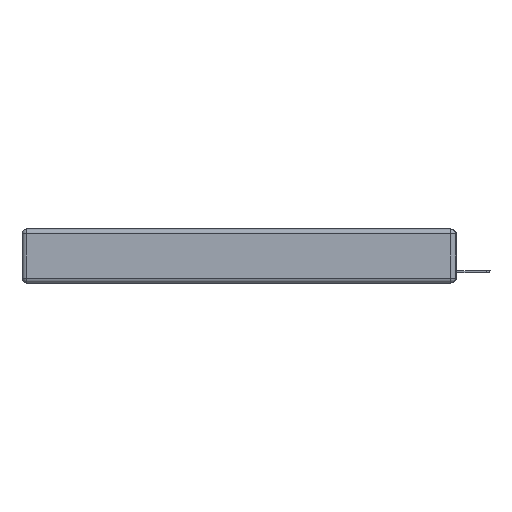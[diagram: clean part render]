
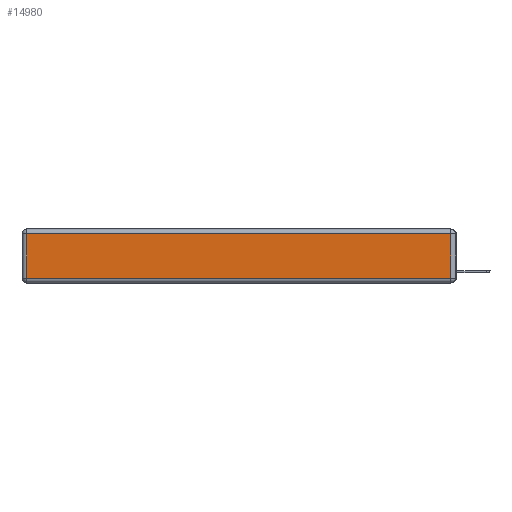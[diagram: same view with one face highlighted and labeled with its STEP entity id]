
A CAD part, left-side view. The second image highlights one B-rep face of the part: STEP entity #14980.
In plain terms, the highlighted planar face has unit normal (-1, 0, 0).
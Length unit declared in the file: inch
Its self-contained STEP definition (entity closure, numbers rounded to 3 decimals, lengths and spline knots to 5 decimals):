
#1404 = LINE ( 'NONE', #7475, #23342 ) ;
#1408 = DIRECTION ( 'NONE',  ( 0., 0., 1. ) ) ;
#1484 = VECTOR ( 'NONE', #13200, 39.37008 ) ;
#1834 = VERTEX_POINT ( 'NONE', #18658 ) ;
#2501 = DIRECTION ( 'NONE',  ( 0., 1., 0. ) ) ;
#3353 = ORIENTED_EDGE ( 'NONE', *, *, #20016, .T. ) ;
#4630 = VERTEX_POINT ( 'NONE', #9718 ) ;
#4944 = FACE_OUTER_BOUND ( 'NONE', #18767, .T. ) ;
#5005 = VECTOR ( 'NONE', #15818, 39.37008 ) ;
#7475 = CARTESIAN_POINT ( 'NONE',  ( 0., 0., -0.313 ) ) ;
#7671 = CARTESIAN_POINT ( 'NONE',  ( 0., 2.75, -0.03 ) ) ;
#8094 = ORIENTED_EDGE ( 'NONE', *, *, #8799, .T. ) ;
#8616 = CARTESIAN_POINT ( 'NONE',  ( 0., 0., -0.343 ) ) ;
#8799 = EDGE_CURVE ( 'NONE', #4630, #20863, #1404, .T. ) ;
#9718 = CARTESIAN_POINT ( 'NONE',  ( 0., 2.72, -0.313 ) ) ;
#12236 = DIRECTION ( 'NONE',  ( -1., 0., 0. ) ) ;
#12781 = VERTEX_POINT ( 'NONE', #13892 ) ;
#13046 = LINE ( 'NONE', #18549, #1484 ) ;
#13200 = DIRECTION ( 'NONE',  ( 0., 0., 1. ) ) ;
#13315 = ORIENTED_EDGE ( 'NONE', *, *, #15921, .T. ) ;
#13892 = CARTESIAN_POINT ( 'NONE',  ( 0., 2.72, -0.03 ) ) ;
#14158 = AXIS2_PLACEMENT_3D ( 'NONE', #8616, #12236, #1408 ) ;
#14569 = DIRECTION ( 'NONE',  ( 0., -1., 0. ) ) ;
#14980 = ADVANCED_FACE ( 'NONE', ( #4944 ), #19555, .T. ) ;
#15818 = DIRECTION ( 'NONE',  ( 0., 0., -1. ) ) ;
#15921 = EDGE_CURVE ( 'NONE', #20863, #1834, #13046, .T. ) ;
#16050 = CARTESIAN_POINT ( 'NONE',  ( 0., 2.72, -0.343 ) ) ;
#18222 = ORIENTED_EDGE ( 'NONE', *, *, #19063, .T. ) ;
#18278 = LINE ( 'NONE', #7671, #18864 ) ;
#18549 = CARTESIAN_POINT ( 'NONE',  ( 0., 0.03, -0.343 ) ) ;
#18658 = CARTESIAN_POINT ( 'NONE',  ( 0., 0.03, -0.03 ) ) ;
#18767 = EDGE_LOOP ( 'NONE', ( #8094, #13315, #18222, #3353 ) ) ;
#18864 = VECTOR ( 'NONE', #2501, 39.37008 ) ;
#19063 = EDGE_CURVE ( 'NONE', #1834, #12781, #18278, .T. ) ;
#19432 = CARTESIAN_POINT ( 'NONE',  ( 0., 0.03, -0.313 ) ) ;
#19555 = PLANE ( 'NONE',  #14158 ) ;
#20016 = EDGE_CURVE ( 'NONE', #12781, #4630, #20827, .T. ) ;
#20827 = LINE ( 'NONE', #16050, #5005 ) ;
#20863 = VERTEX_POINT ( 'NONE', #19432 ) ;
#23342 = VECTOR ( 'NONE', #14569, 39.37008 ) ;
